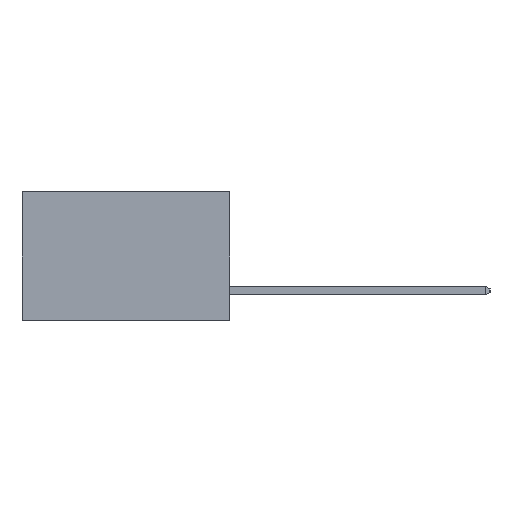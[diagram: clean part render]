
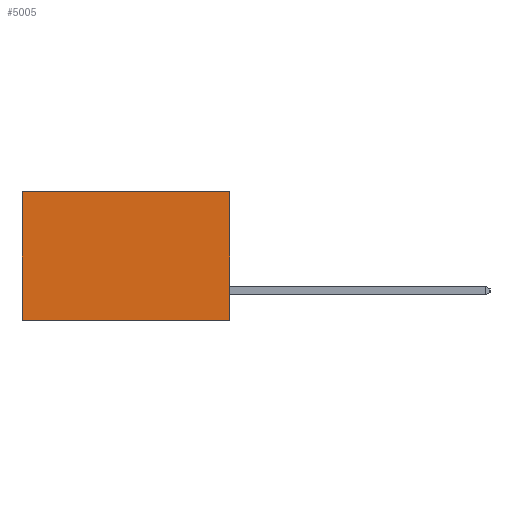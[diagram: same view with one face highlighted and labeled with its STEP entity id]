
A CAD part, left-side view. The second image highlights one B-rep face of the part: STEP entity #5005.
In plain terms, the highlighted planar face has unit normal (-1, 0, 0).
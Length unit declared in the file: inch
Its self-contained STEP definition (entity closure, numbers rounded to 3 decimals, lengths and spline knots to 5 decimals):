
#455 = CARTESIAN_POINT ( 'NONE',  ( 0.2615, 0.6, -0.37 ) ) ;
#812 = LINE ( 'NONE', #8204, #6153 ) ;
#948 = EDGE_CURVE ( 'NONE', #11085, #7111, #812, .T. ) ;
#992 = EDGE_CURVE ( 'NONE', #12319, #11085, #2811, .T. ) ;
#1256 = EDGE_CURVE ( 'NONE', #12319, #7551, #10009, .T. ) ;
#1933 = ORIENTED_EDGE ( 'NONE', *, *, #3897, .T. ) ;
#2316 = ORIENTED_EDGE ( 'NONE', *, *, #948, .F. ) ;
#2697 = ORIENTED_EDGE ( 'NONE', *, *, #992, .F. ) ;
#2811 = LINE ( 'NONE', #9738, #12292 ) ;
#2957 = DIRECTION ( 'NONE',  ( 1., 0., 0. ) ) ;
#3351 = DIRECTION ( 'NONE',  ( 0., 1., 0. ) ) ;
#3352 = AXIS2_PLACEMENT_3D ( 'NONE', #7815, #2957, #9570 ) ;
#3897 = EDGE_CURVE ( 'NONE', #7551, #7111, #6389, .T. ) ;
#4492 = DIRECTION ( 'NONE',  ( 0., 0., -1. ) ) ;
#4789 = CARTESIAN_POINT ( 'NONE',  ( 0.2615, 0., 0. ) ) ;
#4860 = EDGE_LOOP ( 'NONE', ( #1933, #2316, #2697, #8859 ) ) ;
#5005 = ADVANCED_FACE ( 'NONE', ( #10079 ), #6916, .F. ) ;
#5507 = CARTESIAN_POINT ( 'NONE',  ( 0.2615, 0.6, -0.37 ) ) ;
#6153 = VECTOR ( 'NONE', #3351, 39.37008 ) ;
#6389 = LINE ( 'NONE', #5507, #8473 ) ;
#6444 = CARTESIAN_POINT ( 'NONE',  ( 0.2615, 0., 0. ) ) ;
#6916 = PLANE ( 'NONE',  #3352 ) ;
#7111 = VERTEX_POINT ( 'NONE', #455 ) ;
#7551 = VERTEX_POINT ( 'NONE', #10593 ) ;
#7815 = CARTESIAN_POINT ( 'NONE',  ( 0.2615, 0., -0.37 ) ) ;
#8204 = CARTESIAN_POINT ( 'NONE',  ( 0.2615, 0., -0.37 ) ) ;
#8473 = VECTOR ( 'NONE', #4492, 39.37008 ) ;
#8554 = CARTESIAN_POINT ( 'NONE',  ( 0.2615, 0., -0.37 ) ) ;
#8859 = ORIENTED_EDGE ( 'NONE', *, *, #1256, .T. ) ;
#9570 = DIRECTION ( 'NONE',  ( 0., 0., -1. ) ) ;
#9738 = CARTESIAN_POINT ( 'NONE',  ( 0.2615, 0., -0.37 ) ) ;
#9745 = VECTOR ( 'NONE', #10905, 39.37008 ) ;
#10009 = LINE ( 'NONE', #6444, #9745 ) ;
#10079 = FACE_OUTER_BOUND ( 'NONE', #4860, .T. ) ;
#10327 = DIRECTION ( 'NONE',  ( 0., 0., -1. ) ) ;
#10593 = CARTESIAN_POINT ( 'NONE',  ( 0.2615, 0.6, 0. ) ) ;
#10905 = DIRECTION ( 'NONE',  ( 0., 1., 0. ) ) ;
#11085 = VERTEX_POINT ( 'NONE', #8554 ) ;
#12292 = VECTOR ( 'NONE', #10327, 39.37008 ) ;
#12319 = VERTEX_POINT ( 'NONE', #4789 ) ;
